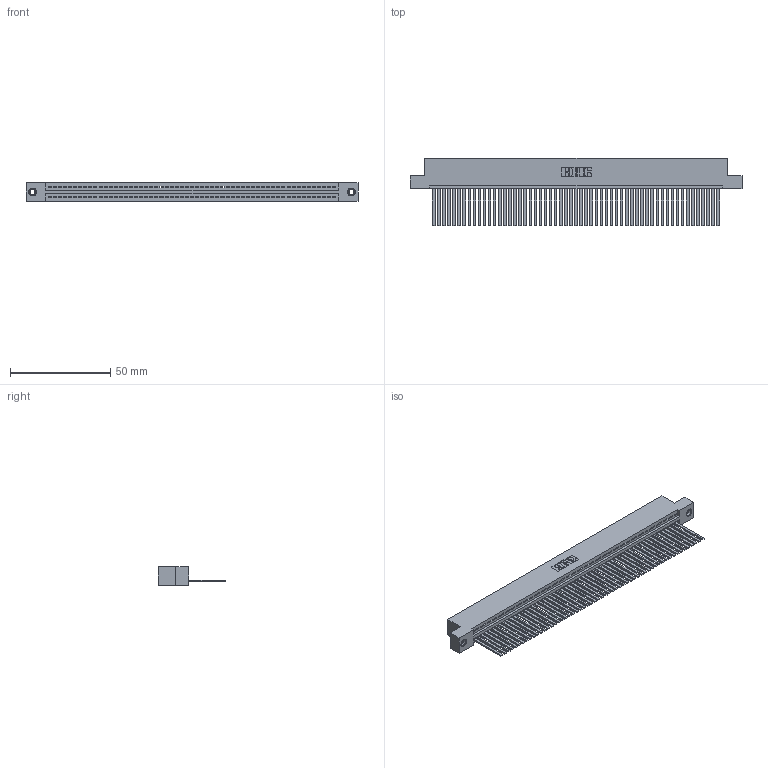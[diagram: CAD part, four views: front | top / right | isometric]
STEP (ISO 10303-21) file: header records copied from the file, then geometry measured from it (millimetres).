
FILE_DESCRIPTION (( 'STEP AP203' ), '1' );
FILE_NAME ('345-057-544-107.STEP', '2019-10-10T14:34:44', ( '' ), ( '' ), 'SwSTEP 2.0', 'SolidWorks 2016', '' );
FILE_SCHEMA (( 'CONFIG_CONTROL_DESIGN' ));
Length unit declared in the file: inch
Products named in the file (4): 345-250-001_345-250-005-103; 345-057-544-107; 345-292-001_345-293-144; 345 Part_Flush Mounting Lugs - 0.156 Dia-TI
Assembly tree (60 placements, depth 2):
  345-057-544-107
    345 Part_Flush Mounting Lugs - 0.156 Dia-TI
    345-292-001_345-293-144  x57
    345-250-001_345-250-005-103  x2
Bounding box: 165.99 x 33.96 x 9.4 mm (x, y, z)
Volume: 16535.3 mm3; surface area: 24192.1 mm2
Topology: 60 solids, 60 shells, 3150 faces, 9483 edges, 6238 vertices
Faces by surface type: plane 2164, cylinder 970, cone 12, torus 4
Entity records: 41882 total; most frequent: CARTESIAN_POINT 7234, ORIENTED_EDGE 7218, DIRECTION 6321, EDGE_CURVE 3609, LINE 3233, VECTOR 3233, VERTEX_POINT 2400, AXIS2_PLACEMENT_3D 1544
